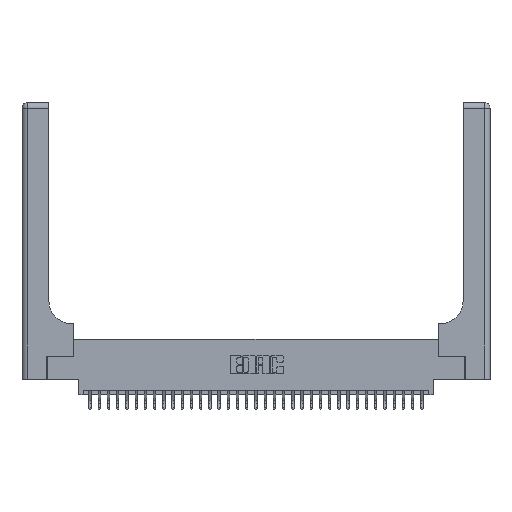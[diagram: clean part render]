
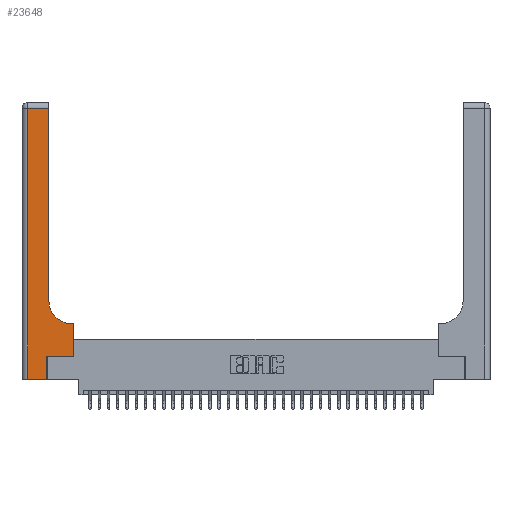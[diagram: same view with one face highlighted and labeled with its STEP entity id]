
A CAD part, top view. The second image highlights one B-rep face of the part: STEP entity #23648.
In plain terms, the highlighted planar face has unit normal (0, 0, 1).
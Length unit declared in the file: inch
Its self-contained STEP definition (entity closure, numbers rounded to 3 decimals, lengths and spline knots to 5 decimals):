
#10 = DIRECTION ( 'NONE',  ( -1., 0., 0. ) ) ;
#89 = CARTESIAN_POINT ( 'NONE',  ( 0.06, 2.94, 0.37 ) ) ;
#125 = CARTESIAN_POINT ( 'NONE',  ( 0.2915, 0.6, 0.37 ) ) ;
#284 = VECTOR ( 'NONE', #1120, 39.37008 ) ;
#290 = DIRECTION ( 'NONE',  ( 0., 1., 0. ) ) ;
#803 = AXIS2_PLACEMENT_3D ( 'NONE', #17792, #6840, #26009 ) ;
#822 = CARTESIAN_POINT ( 'NONE',  ( 0.5585, 0.6, 0.37 ) ) ;
#987 = EDGE_CURVE ( 'NONE', #26435, #17380, #12258, .T. ) ;
#1120 = DIRECTION ( 'NONE',  ( 0., -1., 0. ) ) ;
#2341 = CIRCLE ( 'NONE', #12746, 0.25 ) ;
#2758 = DIRECTION ( 'NONE',  ( 0., 1., 0. ) ) ;
#2810 = ORIENTED_EDGE ( 'NONE', *, *, #20562, .T. ) ;
#3690 = VERTEX_POINT ( 'NONE', #822 ) ;
#4074 = ORIENTED_EDGE ( 'NONE', *, *, #12793, .T. ) ;
#4366 = EDGE_LOOP ( 'NONE', ( #9666, #24252, #4074, #33061, #13172, #27631, #15747, #2810, #24684 ) ) ;
#5786 = DIRECTION ( 'NONE',  ( 0., 1., 0. ) ) ;
#6075 = FACE_OUTER_BOUND ( 'NONE', #4366, .T. ) ;
#6738 = VECTOR ( 'NONE', #31892, 39.37008 ) ;
#6840 = DIRECTION ( 'NONE',  ( 0., 0., -1. ) ) ;
#7314 = VECTOR ( 'NONE', #26082, 39.37008 ) ;
#8587 = EDGE_CURVE ( 'NONE', #26714, #18107, #2341, .T. ) ;
#8671 = DIRECTION ( 'NONE',  ( 0., 0., -1. ) ) ;
#8794 = VERTEX_POINT ( 'NONE', #31777 ) ;
#9505 = VERTEX_POINT ( 'NONE', #10468 ) ;
#9666 = ORIENTED_EDGE ( 'NONE', *, *, #21897, .T. ) ;
#10468 = CARTESIAN_POINT ( 'NONE',  ( 0.06, 0., 0.37 ) ) ;
#11615 = CARTESIAN_POINT ( 'NONE',  ( 0.269, 0.25, 0.37 ) ) ;
#11628 = EDGE_CURVE ( 'NONE', #26402, #8794, #14105, .T. ) ;
#11793 = LINE ( 'NONE', #19208, #32597 ) ;
#12258 = LINE ( 'NONE', #15272, #32216 ) ;
#12746 = AXIS2_PLACEMENT_3D ( 'NONE', #25058, #8671, #27794 ) ;
#12793 = EDGE_CURVE ( 'NONE', #17380, #9505, #28509, .T. ) ;
#13172 = ORIENTED_EDGE ( 'NONE', *, *, #18670, .T. ) ;
#13786 = CARTESIAN_POINT ( 'NONE',  ( 0.2915, 0.85, 0.37 ) ) ;
#14105 = LINE ( 'NONE', #26501, #6738 ) ;
#15129 = CARTESIAN_POINT ( 'NONE',  ( 0.269, 0., 0.37 ) ) ;
#15272 = CARTESIAN_POINT ( 'NONE',  ( 0., 2.94, 0.37 ) ) ;
#15747 = ORIENTED_EDGE ( 'NONE', *, *, #16038, .T. ) ;
#16038 = EDGE_CURVE ( 'NONE', #8794, #3690, #23972, .T. ) ;
#16385 = LINE ( 'NONE', #32947, #22789 ) ;
#17380 = VERTEX_POINT ( 'NONE', #89 ) ;
#17792 = CARTESIAN_POINT ( 'NONE',  ( 0., 3., 0.37 ) ) ;
#18009 = DIRECTION ( 'NONE',  ( -1., 0., 0. ) ) ;
#18107 = VERTEX_POINT ( 'NONE', #13786 ) ;
#18670 = EDGE_CURVE ( 'NONE', #21423, #26402, #11793, .T. ) ;
#19208 = CARTESIAN_POINT ( 'NONE',  ( 0.269, 0., 0.37 ) ) ;
#19970 = CARTESIAN_POINT ( 'NONE',  ( 0.2915, 2.94, 0.37 ) ) ;
#20562 = EDGE_CURVE ( 'NONE', #3690, #26714, #26183, .T. ) ;
#20722 = CARTESIAN_POINT ( 'NONE',  ( 0.06, 3., 0.37 ) ) ;
#21423 = VERTEX_POINT ( 'NONE', #15129 ) ;
#21897 = EDGE_CURVE ( 'NONE', #18107, #26435, #16385, .T. ) ;
#22789 = VECTOR ( 'NONE', #290, 39.37008 ) ;
#23290 = PLANE ( 'NONE',  #803 ) ;
#23648 = ADVANCED_FACE ( 'NONE', ( #6075 ), #23290, .F. ) ;
#23972 = LINE ( 'NONE', #27659, #30302 ) ;
#24252 = ORIENTED_EDGE ( 'NONE', *, *, #987, .T. ) ;
#24265 = CARTESIAN_POINT ( 'NONE',  ( 0.5415, 0.6, 0.37 ) ) ;
#24684 = ORIENTED_EDGE ( 'NONE', *, *, #8587, .T. ) ;
#25058 = CARTESIAN_POINT ( 'NONE',  ( 0.5415, 0.85, 0.37 ) ) ;
#26009 = DIRECTION ( 'NONE',  ( -1., 0., 0. ) ) ;
#26082 = DIRECTION ( 'NONE',  ( 1., 0., 0. ) ) ;
#26183 = LINE ( 'NONE', #125, #32467 ) ;
#26402 = VERTEX_POINT ( 'NONE', #11615 ) ;
#26435 = VERTEX_POINT ( 'NONE', #19970 ) ;
#26501 = CARTESIAN_POINT ( 'NONE',  ( 0.269, 0.25, 0.37 ) ) ;
#26714 = VERTEX_POINT ( 'NONE', #24265 ) ;
#27631 = ORIENTED_EDGE ( 'NONE', *, *, #11628, .T. ) ;
#27659 = CARTESIAN_POINT ( 'NONE',  ( 0.5585, 0.25, 0.37 ) ) ;
#27794 = DIRECTION ( 'NONE',  ( 1., 0., 0. ) ) ;
#28509 = LINE ( 'NONE', #20722, #284 ) ;
#28762 = CARTESIAN_POINT ( 'NONE',  ( 0., 0., 0.37 ) ) ;
#29113 = LINE ( 'NONE', #28762, #7314 ) ;
#30302 = VECTOR ( 'NONE', #5786, 39.37008 ) ;
#31777 = CARTESIAN_POINT ( 'NONE',  ( 0.5585, 0.25, 0.37 ) ) ;
#31892 = DIRECTION ( 'NONE',  ( 1., 0., 0. ) ) ;
#32216 = VECTOR ( 'NONE', #18009, 39.37008 ) ;
#32467 = VECTOR ( 'NONE', #10, 39.37008 ) ;
#32597 = VECTOR ( 'NONE', #2758, 39.37008 ) ;
#32947 = CARTESIAN_POINT ( 'NONE',  ( 0.2915, 3., 0.37 ) ) ;
#33061 = ORIENTED_EDGE ( 'NONE', *, *, #33750, .T. ) ;
#33750 = EDGE_CURVE ( 'NONE', #9505, #21423, #29113, .T. ) ;
